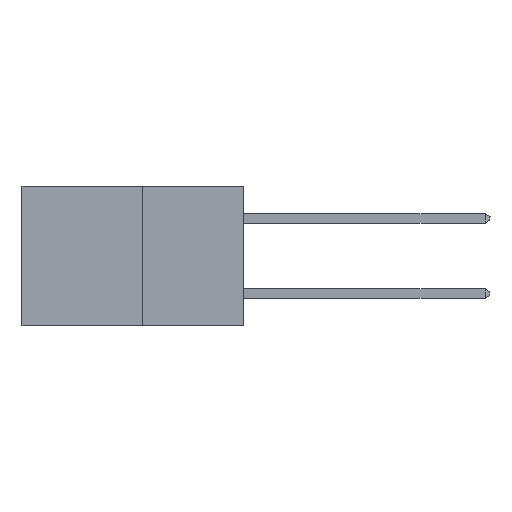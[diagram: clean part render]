
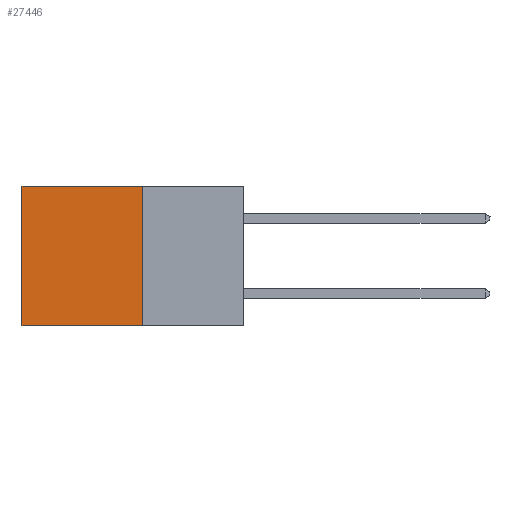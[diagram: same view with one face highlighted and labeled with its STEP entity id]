
A CAD part, left-side view. The second image highlights one B-rep face of the part: STEP entity #27446.
In plain terms, the highlighted planar face has unit normal (-1, 0, 0).
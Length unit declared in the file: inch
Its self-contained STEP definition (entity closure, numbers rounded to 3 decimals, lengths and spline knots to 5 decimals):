
#1187 = CARTESIAN_POINT ( 'NONE',  ( 0.277, 0.27, 0. ) ) ;
#2165 = CARTESIAN_POINT ( 'NONE',  ( 0.277, 0.27, -0.37 ) ) ;
#2327 = LINE ( 'NONE', #2165, #14751 ) ;
#2456 = VERTEX_POINT ( 'NONE', #21586 ) ;
#2501 = DIRECTION ( 'NONE',  ( 1., 0., 0. ) ) ;
#2828 = ORIENTED_EDGE ( 'NONE', *, *, #22838, .F. ) ;
#4632 = DIRECTION ( 'NONE',  ( 0., 0., -1. ) ) ;
#4830 = CARTESIAN_POINT ( 'NONE',  ( 0.277, 0.59, 0. ) ) ;
#7779 = ORIENTED_EDGE ( 'NONE', *, *, #24869, .T. ) ;
#10694 = VECTOR ( 'NONE', #31431, 39.37008 ) ;
#10852 = VERTEX_POINT ( 'NONE', #4830 ) ;
#11020 = CARTESIAN_POINT ( 'NONE',  ( 0.277, 0.59, -0.37 ) ) ;
#11065 = CARTESIAN_POINT ( 'NONE',  ( 0.277, 0.27, -0.37 ) ) ;
#11883 = EDGE_CURVE ( 'NONE', #2456, #21007, #20523, .T. ) ;
#13330 = FACE_OUTER_BOUND ( 'NONE', #24156, .T. ) ;
#13829 = LINE ( 'NONE', #31817, #19735 ) ;
#14751 = VECTOR ( 'NONE', #4632, 39.37008 ) ;
#16669 = ORIENTED_EDGE ( 'NONE', *, *, #11883, .F. ) ;
#17394 = CARTESIAN_POINT ( 'NONE',  ( 0.277, 0.27, -0.37 ) ) ;
#18551 = ORIENTED_EDGE ( 'NONE', *, *, #25879, .T. ) ;
#18653 = DIRECTION ( 'NONE',  ( 0., 1., 0. ) ) ;
#19585 = DIRECTION ( 'NONE',  ( 0., 0., -1. ) ) ;
#19725 = VECTOR ( 'NONE', #18653, 39.37008 ) ;
#19735 = VECTOR ( 'NONE', #19585, 39.37008 ) ;
#19941 = DIRECTION ( 'NONE',  ( 0., 0., -1. ) ) ;
#20523 = LINE ( 'NONE', #11065, #19725 ) ;
#20675 = AXIS2_PLACEMENT_3D ( 'NONE', #17394, #2501, #19941 ) ;
#21007 = VERTEX_POINT ( 'NONE', #11020 ) ;
#21586 = CARTESIAN_POINT ( 'NONE',  ( 0.277, 0.27, -0.37 ) ) ;
#22681 = VERTEX_POINT ( 'NONE', #1187 ) ;
#22838 = EDGE_CURVE ( 'NONE', #22681, #2456, #2327, .T. ) ;
#24156 = EDGE_LOOP ( 'NONE', ( #18551, #16669, #2828, #7779 ) ) ;
#24869 = EDGE_CURVE ( 'NONE', #22681, #10852, #30526, .T. ) ;
#25879 = EDGE_CURVE ( 'NONE', #10852, #21007, #13829, .T. ) ;
#27446 = ADVANCED_FACE ( 'NONE', ( #13330 ), #32055, .F. ) ;
#29015 = CARTESIAN_POINT ( 'NONE',  ( 0.277, 0.27, 0. ) ) ;
#30526 = LINE ( 'NONE', #29015, #10694 ) ;
#31431 = DIRECTION ( 'NONE',  ( 0., 1., 0. ) ) ;
#31817 = CARTESIAN_POINT ( 'NONE',  ( 0.277, 0.59, -0.37 ) ) ;
#32055 = PLANE ( 'NONE',  #20675 ) ;
